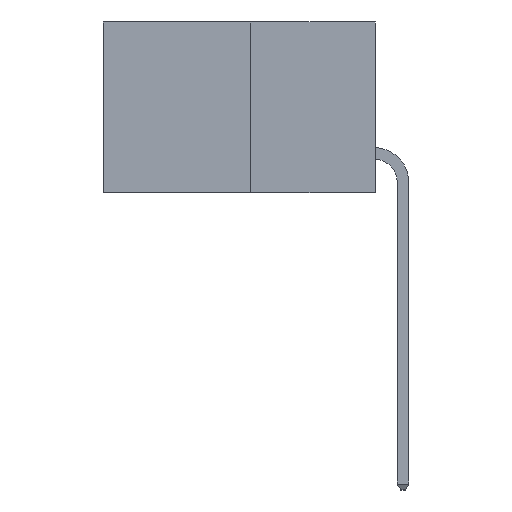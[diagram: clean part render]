
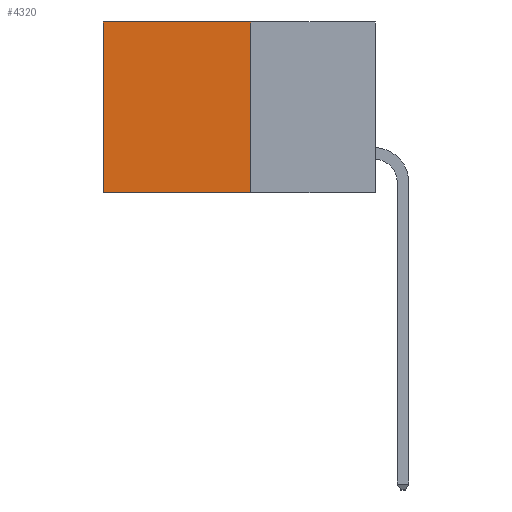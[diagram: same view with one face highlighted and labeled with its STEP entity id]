
A CAD part, left-side view. The second image highlights one B-rep face of the part: STEP entity #4320.
In plain terms, the highlighted planar face has unit normal (-1, 0, 0).
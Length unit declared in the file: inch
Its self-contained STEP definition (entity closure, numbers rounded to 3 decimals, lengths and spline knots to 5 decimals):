
#804 = EDGE_LOOP ( 'NONE', ( #3824, #9082, #8822, #2489 ) ) ;
#907 = CARTESIAN_POINT ( 'NONE',  ( 0.277, 0.27, 0. ) ) ;
#1512 = LINE ( 'NONE', #907, #5467 ) ;
#1614 = LINE ( 'NONE', #1654, #1869 ) ;
#1654 = CARTESIAN_POINT ( 'NONE',  ( 0.277, 0.59, -0.37 ) ) ;
#1756 = EDGE_CURVE ( 'NONE', #6092, #5240, #1614, .T. ) ;
#1848 = VECTOR ( 'NONE', #3902, 39.37008 ) ;
#1869 = VECTOR ( 'NONE', #3959, 39.37008 ) ;
#2054 = AXIS2_PLACEMENT_3D ( 'NONE', #5279, #5265, #5254 ) ;
#2489 = ORIENTED_EDGE ( 'NONE', *, *, #6811, .T. ) ;
#2513 = EDGE_CURVE ( 'NONE', #4336, #5240, #7422, .T. ) ;
#2670 = EDGE_CURVE ( 'NONE', #5507, #4336, #3956, .T. ) ;
#2975 = CARTESIAN_POINT ( 'NONE',  ( 0.277, 0.59, -0.37 ) ) ;
#3279 = CARTESIAN_POINT ( 'NONE',  ( 0.277, 0.27, 0. ) ) ;
#3496 = CARTESIAN_POINT ( 'NONE',  ( 0.277, 0.27, -0.37 ) ) ;
#3824 = ORIENTED_EDGE ( 'NONE', *, *, #1756, .T. ) ;
#3828 = CARTESIAN_POINT ( 'NONE',  ( 0.277, 0.27, -0.37 ) ) ;
#3902 = DIRECTION ( 'NONE',  ( 0., 0., -1. ) ) ;
#3956 = LINE ( 'NONE', #3828, #1848 ) ;
#3959 = DIRECTION ( 'NONE',  ( 0., 0., -1. ) ) ;
#4320 = ADVANCED_FACE ( 'NONE', ( #7389 ), #5289, .F. ) ;
#4336 = VERTEX_POINT ( 'NONE', #5148 ) ;
#5148 = CARTESIAN_POINT ( 'NONE',  ( 0.277, 0.27, -0.37 ) ) ;
#5240 = VERTEX_POINT ( 'NONE', #2975 ) ;
#5254 = DIRECTION ( 'NONE',  ( 0., 0., -1. ) ) ;
#5265 = DIRECTION ( 'NONE',  ( 1., 0., 0. ) ) ;
#5279 = CARTESIAN_POINT ( 'NONE',  ( 0.277, 0.27, -0.37 ) ) ;
#5289 = PLANE ( 'NONE',  #2054 ) ;
#5467 = VECTOR ( 'NONE', #9369, 39.37008 ) ;
#5507 = VERTEX_POINT ( 'NONE', #3279 ) ;
#6092 = VERTEX_POINT ( 'NONE', #9288 ) ;
#6338 = DIRECTION ( 'NONE',  ( 0., 1., 0. ) ) ;
#6811 = EDGE_CURVE ( 'NONE', #5507, #6092, #1512, .T. ) ;
#7389 = FACE_OUTER_BOUND ( 'NONE', #804, .T. ) ;
#7422 = LINE ( 'NONE', #3496, #9146 ) ;
#8822 = ORIENTED_EDGE ( 'NONE', *, *, #2670, .F. ) ;
#9082 = ORIENTED_EDGE ( 'NONE', *, *, #2513, .F. ) ;
#9146 = VECTOR ( 'NONE', #6338, 39.37008 ) ;
#9288 = CARTESIAN_POINT ( 'NONE',  ( 0.277, 0.59, 0. ) ) ;
#9369 = DIRECTION ( 'NONE',  ( 0., 1., 0. ) ) ;
